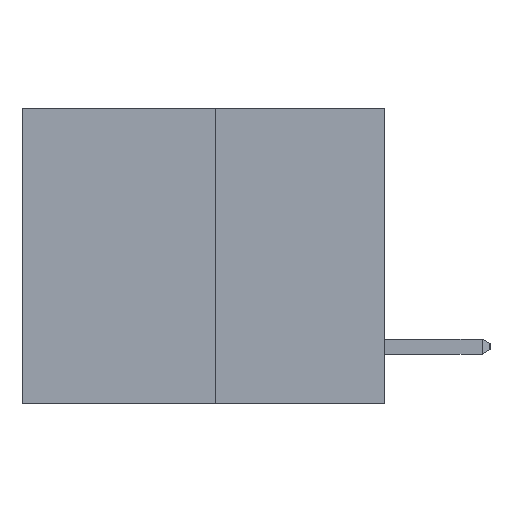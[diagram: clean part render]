
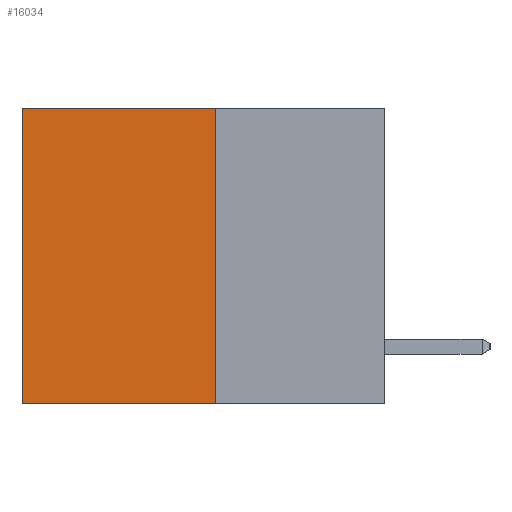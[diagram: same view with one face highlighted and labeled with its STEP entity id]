
A CAD part, left-side view. The second image highlights one B-rep face of the part: STEP entity #16034.
In plain terms, the highlighted planar face has unit normal (-1, 0, 0).
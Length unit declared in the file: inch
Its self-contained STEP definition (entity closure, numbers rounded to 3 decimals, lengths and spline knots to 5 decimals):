
#95 = EDGE_LOOP ( 'NONE', ( #8680, #114, #19722, #539 ) ) ;
#99 = EDGE_CURVE ( 'NONE', #7528, #14060, #983, .T. ) ;
#114 = ORIENTED_EDGE ( 'NONE', *, *, #4650, .F. ) ;
#539 = ORIENTED_EDGE ( 'NONE', *, *, #99, .T. ) ;
#796 = AXIS2_PLACEMENT_3D ( 'NONE', #11995, #14144, #22863 ) ;
#983 = LINE ( 'NONE', #20479, #18630 ) ;
#1030 = PLANE ( 'NONE',  #796 ) ;
#2986 = DIRECTION ( 'NONE',  ( 0., 1., 0. ) ) ;
#3664 = LINE ( 'NONE', #22694, #5717 ) ;
#4650 = EDGE_CURVE ( 'NONE', #11531, #6770, #26558, .T. ) ;
#5717 = VECTOR ( 'NONE', #14455, 39.37008 ) ;
#6770 = VERTEX_POINT ( 'NONE', #15159 ) ;
#7528 = VERTEX_POINT ( 'NONE', #25304 ) ;
#8105 = CARTESIAN_POINT ( 'NONE',  ( 0.3165, 0.28, -0.49 ) ) ;
#8680 = ORIENTED_EDGE ( 'NONE', *, *, #10752, .T. ) ;
#10752 = EDGE_CURVE ( 'NONE', #14060, #6770, #3664, .T. ) ;
#11294 = VECTOR ( 'NONE', #11999, 39.37008 ) ;
#11531 = VERTEX_POINT ( 'NONE', #18532 ) ;
#11995 = CARTESIAN_POINT ( 'NONE',  ( 0.3165, 0.28, -0.49 ) ) ;
#11999 = DIRECTION ( 'NONE',  ( 0., 0., -1. ) ) ;
#14060 = VERTEX_POINT ( 'NONE', #15545 ) ;
#14144 = DIRECTION ( 'NONE',  ( 1., 0., 0. ) ) ;
#14455 = DIRECTION ( 'NONE',  ( 0., 0., -1. ) ) ;
#15159 = CARTESIAN_POINT ( 'NONE',  ( 0.3165, 0.6, -0.49 ) ) ;
#15545 = CARTESIAN_POINT ( 'NONE',  ( 0.3165, 0.6, 0. ) ) ;
#15991 = CARTESIAN_POINT ( 'NONE',  ( 0.3165, 0.28, -0.49 ) ) ;
#16034 = ADVANCED_FACE ( 'NONE', ( #23031 ), #1030, .F. ) ;
#18532 = CARTESIAN_POINT ( 'NONE',  ( 0.3165, 0.28, -0.49 ) ) ;
#18630 = VECTOR ( 'NONE', #24875, 39.37008 ) ;
#19722 = ORIENTED_EDGE ( 'NONE', *, *, #27706, .F. ) ;
#20479 = CARTESIAN_POINT ( 'NONE',  ( 0.3165, 0.28, 0. ) ) ;
#22694 = CARTESIAN_POINT ( 'NONE',  ( 0.3165, 0.6, -0.49 ) ) ;
#22863 = DIRECTION ( 'NONE',  ( 0., 0., -1. ) ) ;
#23031 = FACE_OUTER_BOUND ( 'NONE', #95, .T. ) ;
#24171 = LINE ( 'NONE', #8105, #11294 ) ;
#24875 = DIRECTION ( 'NONE',  ( 0., 1., 0. ) ) ;
#25304 = CARTESIAN_POINT ( 'NONE',  ( 0.3165, 0.28, 0. ) ) ;
#25866 = VECTOR ( 'NONE', #2986, 39.37008 ) ;
#26558 = LINE ( 'NONE', #15991, #25866 ) ;
#27706 = EDGE_CURVE ( 'NONE', #7528, #11531, #24171, .T. ) ;
